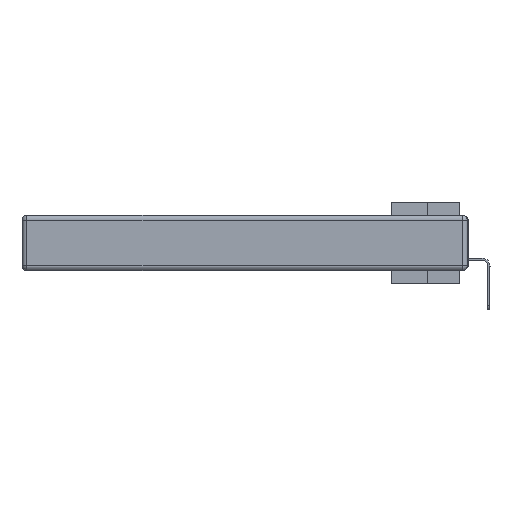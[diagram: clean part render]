
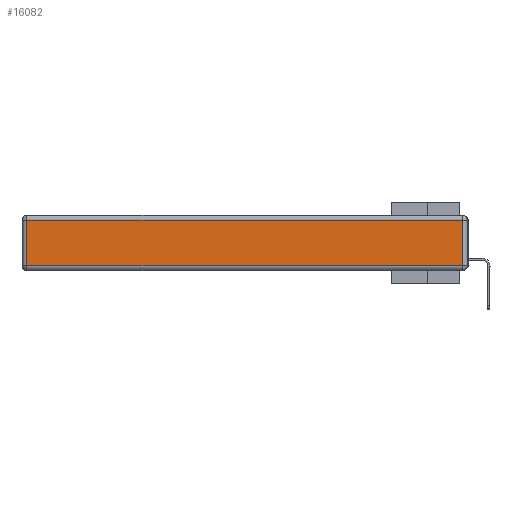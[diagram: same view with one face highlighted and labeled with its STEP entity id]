
A CAD part, left-side view. The second image highlights one B-rep face of the part: STEP entity #16082.
In plain terms, the highlighted planar face has unit normal (-1, 0, 0).
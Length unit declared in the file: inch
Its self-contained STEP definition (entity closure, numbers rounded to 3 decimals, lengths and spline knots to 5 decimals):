
#1998 = EDGE_CURVE ( 'NONE', #18173, #29955, #13729, .T. ) ;
#3283 = LINE ( 'NONE', #25422, #13296 ) ;
#3434 = CARTESIAN_POINT ( 'NONE',  ( 0., 0.03, -0.313 ) ) ;
#3910 = DIRECTION ( 'NONE',  ( 0., 0., 1. ) ) ;
#8760 = DIRECTION ( 'NONE',  ( -1., 0., 0. ) ) ;
#9562 = DIRECTION ( 'NONE',  ( 0., 1., 0. ) ) ;
#11139 = DIRECTION ( 'NONE',  ( 0., 0., -1. ) ) ;
#11480 = CARTESIAN_POINT ( 'NONE',  ( 0., 0.03, -0.343 ) ) ;
#11844 = LINE ( 'NONE', #21315, #23782 ) ;
#13030 = AXIS2_PLACEMENT_3D ( 'NONE', #22915, #8760, #3910 ) ;
#13296 = VECTOR ( 'NONE', #11139, 39.37008 ) ;
#13729 = LINE ( 'NONE', #23833, #18578 ) ;
#16082 = ADVANCED_FACE ( 'NONE', ( #20735 ), #18130, .T. ) ;
#16376 = DIRECTION ( 'NONE',  ( 0., 0., 1. ) ) ;
#17061 = VECTOR ( 'NONE', #16376, 39.37008 ) ;
#18130 = PLANE ( 'NONE',  #13030 ) ;
#18173 = VERTEX_POINT ( 'NONE', #23121 ) ;
#18578 = VECTOR ( 'NONE', #9562, 39.37008 ) ;
#18936 = VERTEX_POINT ( 'NONE', #26920 ) ;
#19726 = ORIENTED_EDGE ( 'NONE', *, *, #21081, .T. ) ;
#20735 = FACE_OUTER_BOUND ( 'NONE', #29426, .T. ) ;
#21081 = EDGE_CURVE ( 'NONE', #29906, #18173, #23408, .T. ) ;
#21206 = DIRECTION ( 'NONE',  ( 0., -1., 0. ) ) ;
#21315 = CARTESIAN_POINT ( 'NONE',  ( 0., 0., -0.313 ) ) ;
#21528 = EDGE_CURVE ( 'NONE', #29955, #18936, #3283, .T. ) ;
#21856 = ORIENTED_EDGE ( 'NONE', *, *, #21528, .T. ) ;
#22915 = CARTESIAN_POINT ( 'NONE',  ( 0., 0., -0.343 ) ) ;
#23121 = CARTESIAN_POINT ( 'NONE',  ( 0., 0.03, -0.03 ) ) ;
#23408 = LINE ( 'NONE', #11480, #17061 ) ;
#23418 = ORIENTED_EDGE ( 'NONE', *, *, #27713, .T. ) ;
#23782 = VECTOR ( 'NONE', #21206, 39.37008 ) ;
#23833 = CARTESIAN_POINT ( 'NONE',  ( 0., 2.75, -0.03 ) ) ;
#24003 = ORIENTED_EDGE ( 'NONE', *, *, #1998, .T. ) ;
#25422 = CARTESIAN_POINT ( 'NONE',  ( 0., 2.72, -0.343 ) ) ;
#26920 = CARTESIAN_POINT ( 'NONE',  ( 0., 2.72, -0.313 ) ) ;
#27542 = CARTESIAN_POINT ( 'NONE',  ( 0., 2.72, -0.03 ) ) ;
#27713 = EDGE_CURVE ( 'NONE', #18936, #29906, #11844, .T. ) ;
#29426 = EDGE_LOOP ( 'NONE', ( #23418, #19726, #24003, #21856 ) ) ;
#29906 = VERTEX_POINT ( 'NONE', #3434 ) ;
#29955 = VERTEX_POINT ( 'NONE', #27542 ) ;
